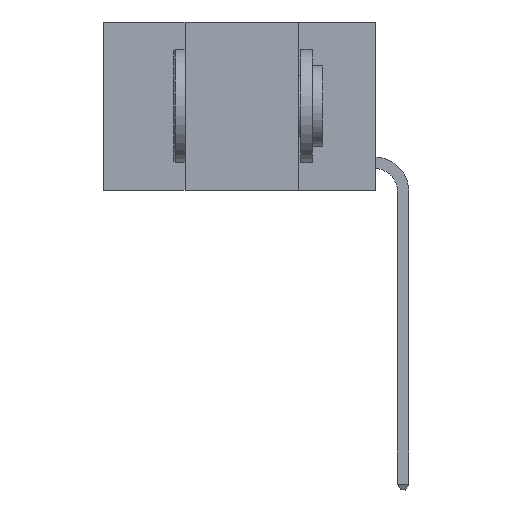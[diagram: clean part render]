
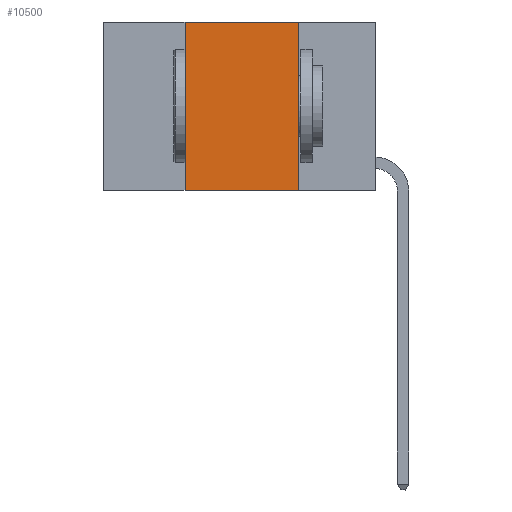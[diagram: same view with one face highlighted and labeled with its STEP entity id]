
A CAD part, left-side view. The second image highlights one B-rep face of the part: STEP entity #10500.
In plain terms, the highlighted planar face has unit normal (-1, 0, 0).
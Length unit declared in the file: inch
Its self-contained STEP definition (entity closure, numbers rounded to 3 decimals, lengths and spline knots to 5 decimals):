
#223 = AXIS2_PLACEMENT_3D ( 'NONE', #1661, #17312, #3905 ) ;
#351 = ORIENTED_EDGE ( 'NONE', *, *, #10091, .F. ) ;
#1661 = CARTESIAN_POINT ( 'NONE',  ( 0., 0.6, 0. ) ) ;
#2924 = FACE_OUTER_BOUND ( 'NONE', #27639, .T. ) ;
#3583 = LINE ( 'NONE', #24979, #14742 ) ;
#3905 = DIRECTION ( 'NONE',  ( 0., 0., -1. ) ) ;
#5610 = CARTESIAN_POINT ( 'NONE',  ( 0., 0.6, -0.37 ) ) ;
#5618 = ORIENTED_EDGE ( 'NONE', *, *, #9440, .F. ) ;
#6588 = VECTOR ( 'NONE', #21228, 39.37008 ) ;
#7403 = CARTESIAN_POINT ( 'NONE',  ( 0., 0.17, -0.37 ) ) ;
#8491 = CARTESIAN_POINT ( 'NONE',  ( 0., 0.42, 0. ) ) ;
#8605 = CARTESIAN_POINT ( 'NONE',  ( 0., 0.17, 0. ) ) ;
#9062 = DIRECTION ( 'NONE',  ( 0., -1., 0. ) ) ;
#9370 = VERTEX_POINT ( 'NONE', #8605 ) ;
#9440 = EDGE_CURVE ( 'NONE', #9370, #19267, #19790, .T. ) ;
#10091 = EDGE_CURVE ( 'NONE', #12575, #9370, #26652, .T. ) ;
#10500 = ADVANCED_FACE ( 'NONE', ( #2924 ), #26123, .F. ) ;
#12575 = VERTEX_POINT ( 'NONE', #8491 ) ;
#13163 = VERTEX_POINT ( 'NONE', #17216 ) ;
#13229 = DIRECTION ( 'NONE',  ( 0., 0., -1. ) ) ;
#13648 = ORIENTED_EDGE ( 'NONE', *, *, #20631, .T. ) ;
#13813 = VECTOR ( 'NONE', #13229, 39.37008 ) ;
#14742 = VECTOR ( 'NONE', #27201, 39.37008 ) ;
#14818 = VECTOR ( 'NONE', #9062, 39.37008 ) ;
#15457 = CARTESIAN_POINT ( 'NONE',  ( 0., 0.17, 0. ) ) ;
#16322 = LINE ( 'NONE', #5610, #6588 ) ;
#17216 = CARTESIAN_POINT ( 'NONE',  ( 0., 0.42, -0.37 ) ) ;
#17312 = DIRECTION ( 'NONE',  ( 1., 0., 0. ) ) ;
#17902 = EDGE_CURVE ( 'NONE', #13163, #12575, #3583, .T. ) ;
#18920 = ORIENTED_EDGE ( 'NONE', *, *, #17902, .F. ) ;
#19267 = VERTEX_POINT ( 'NONE', #7403 ) ;
#19790 = LINE ( 'NONE', #15457, #13813 ) ;
#20245 = CARTESIAN_POINT ( 'NONE',  ( 0., 0.6, 0. ) ) ;
#20631 = EDGE_CURVE ( 'NONE', #13163, #19267, #16322, .T. ) ;
#21228 = DIRECTION ( 'NONE',  ( 0., -1., 0. ) ) ;
#24979 = CARTESIAN_POINT ( 'NONE',  ( 0., 0.42, 0. ) ) ;
#26123 = PLANE ( 'NONE',  #223 ) ;
#26652 = LINE ( 'NONE', #20245, #14818 ) ;
#27201 = DIRECTION ( 'NONE',  ( 0., 0., 1. ) ) ;
#27639 = EDGE_LOOP ( 'NONE', ( #5618, #351, #18920, #13648 ) ) ;
